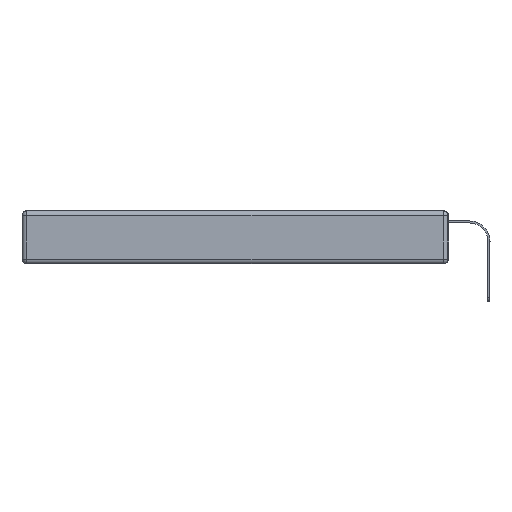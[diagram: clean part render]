
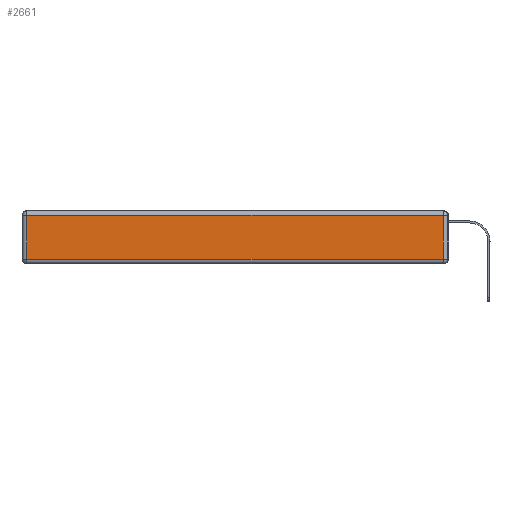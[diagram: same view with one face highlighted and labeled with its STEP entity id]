
A CAD part, left-side view. The second image highlights one B-rep face of the part: STEP entity #2661.
In plain terms, the highlighted planar face has unit normal (-1, 0, 0).
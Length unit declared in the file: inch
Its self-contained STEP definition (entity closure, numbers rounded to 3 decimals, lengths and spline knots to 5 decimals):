
#290 = VECTOR ( 'NONE', #4223, 39.37008 ) ;
#767 = CARTESIAN_POINT ( 'NONE',  ( 0., 0., -0.313 ) ) ;
#1024 = EDGE_CURVE ( 'NONE', #9103, #17170, #12142, .T. ) ;
#1333 = CARTESIAN_POINT ( 'NONE',  ( 0., 0.03, -0.03 ) ) ;
#1528 = FACE_OUTER_BOUND ( 'NONE', #8068, .T. ) ;
#2401 = LINE ( 'NONE', #11024, #15814 ) ;
#2447 = EDGE_CURVE ( 'NONE', #6045, #9103, #2834, .T. ) ;
#2574 = EDGE_CURVE ( 'NONE', #10782, #6045, #5116, .T. ) ;
#2661 = ADVANCED_FACE ( 'NONE', ( #1528 ), #5665, .T. ) ;
#2834 = LINE ( 'NONE', #11258, #290 ) ;
#2869 = ORIENTED_EDGE ( 'NONE', *, *, #2574, .T. ) ;
#4223 = DIRECTION ( 'NONE',  ( 0., 0., -1. ) ) ;
#5116 = LINE ( 'NONE', #13551, #14787 ) ;
#5392 = DIRECTION ( 'NONE',  ( -1., 0., 0. ) ) ;
#5665 = PLANE ( 'NONE',  #15994 ) ;
#6045 = VERTEX_POINT ( 'NONE', #10810 ) ;
#6205 = ORIENTED_EDGE ( 'NONE', *, *, #1024, .T. ) ;
#6392 = DIRECTION ( 'NONE',  ( 0., -1., 0. ) ) ;
#6491 = DIRECTION ( 'NONE',  ( 0., 1., 0. ) ) ;
#8059 = DIRECTION ( 'NONE',  ( 0., 0., 1. ) ) ;
#8068 = EDGE_LOOP ( 'NONE', ( #6205, #12151, #2869, #15895 ) ) ;
#9103 = VERTEX_POINT ( 'NONE', #10034 ) ;
#9748 = CARTESIAN_POINT ( 'NONE',  ( 0., 0.03, -0.313 ) ) ;
#10034 = CARTESIAN_POINT ( 'NONE',  ( 0., 2.72, -0.313 ) ) ;
#10782 = VERTEX_POINT ( 'NONE', #1333 ) ;
#10810 = CARTESIAN_POINT ( 'NONE',  ( 0., 2.72, -0.03 ) ) ;
#11024 = CARTESIAN_POINT ( 'NONE',  ( 0., 0.03, -0.343 ) ) ;
#11070 = EDGE_CURVE ( 'NONE', #17170, #10782, #2401, .T. ) ;
#11258 = CARTESIAN_POINT ( 'NONE',  ( 0., 2.72, -0.343 ) ) ;
#12142 = LINE ( 'NONE', #767, #14836 ) ;
#12151 = ORIENTED_EDGE ( 'NONE', *, *, #11070, .T. ) ;
#12909 = CARTESIAN_POINT ( 'NONE',  ( 0., 0., -0.343 ) ) ;
#13551 = CARTESIAN_POINT ( 'NONE',  ( 0., 2.75, -0.03 ) ) ;
#14787 = VECTOR ( 'NONE', #6491, 39.37008 ) ;
#14836 = VECTOR ( 'NONE', #6392, 39.37008 ) ;
#15524 = DIRECTION ( 'NONE',  ( 0., 0., 1. ) ) ;
#15814 = VECTOR ( 'NONE', #8059, 39.37008 ) ;
#15895 = ORIENTED_EDGE ( 'NONE', *, *, #2447, .T. ) ;
#15994 = AXIS2_PLACEMENT_3D ( 'NONE', #12909, #5392, #15524 ) ;
#17170 = VERTEX_POINT ( 'NONE', #9748 ) ;
